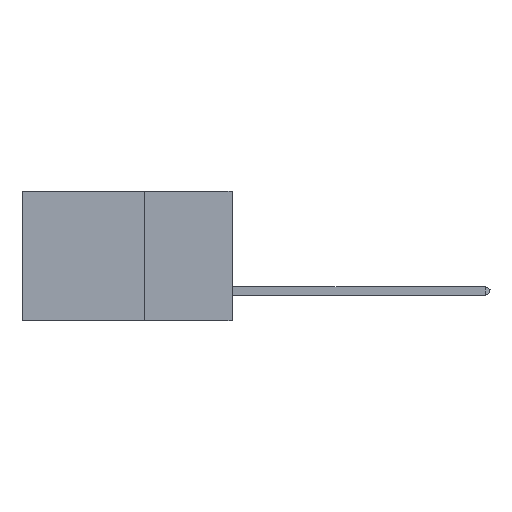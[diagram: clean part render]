
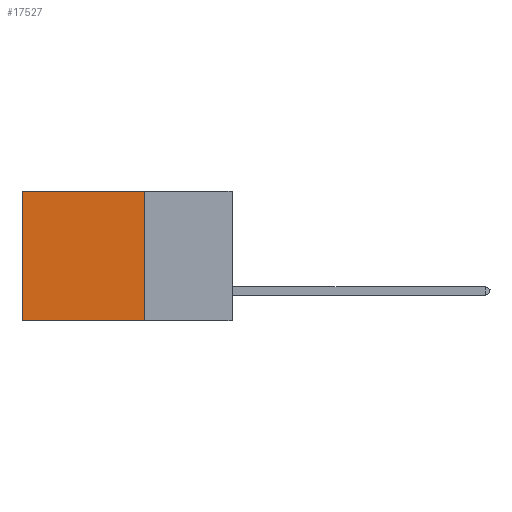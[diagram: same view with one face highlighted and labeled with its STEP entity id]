
A CAD part, left-side view. The second image highlights one B-rep face of the part: STEP entity #17527.
In plain terms, the highlighted planar face has unit normal (-1, 0, 0).
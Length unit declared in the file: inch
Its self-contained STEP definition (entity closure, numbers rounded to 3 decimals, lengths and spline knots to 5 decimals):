
#637 = CARTESIAN_POINT ( 'NONE',  ( 0.2875, 0.6, 0. ) ) ;
#1675 = VECTOR ( 'NONE', #4019, 39.37008 ) ;
#2315 = ORIENTED_EDGE ( 'NONE', *, *, #25332, .F. ) ;
#2528 = DIRECTION ( 'NONE',  ( 0., 1., 0. ) ) ;
#3520 = EDGE_CURVE ( 'NONE', #17088, #13766, #10512, .T. ) ;
#3753 = ORIENTED_EDGE ( 'NONE', *, *, #3520, .T. ) ;
#4019 = DIRECTION ( 'NONE',  ( 0., 1., 0. ) ) ;
#4047 = DIRECTION ( 'NONE',  ( 0., 0., -1. ) ) ;
#4694 = DIRECTION ( 'NONE',  ( 0., 0., -1. ) ) ;
#7903 = VECTOR ( 'NONE', #2528, 39.37008 ) ;
#8524 = VERTEX_POINT ( 'NONE', #17369 ) ;
#9736 = LINE ( 'NONE', #20987, #1675 ) ;
#10512 = LINE ( 'NONE', #12721, #28768 ) ;
#11515 = LINE ( 'NONE', #21692, #14612 ) ;
#12721 = CARTESIAN_POINT ( 'NONE',  ( 0.2875, 0.6, 0. ) ) ;
#13766 = VERTEX_POINT ( 'NONE', #29710 ) ;
#14612 = VECTOR ( 'NONE', #4694, 39.37008 ) ;
#16656 = FACE_OUTER_BOUND ( 'NONE', #34417, .T. ) ;
#17088 = VERTEX_POINT ( 'NONE', #637 ) ;
#17369 = CARTESIAN_POINT ( 'NONE',  ( 0.2875, 0.25, -0.37 ) ) ;
#17527 = ADVANCED_FACE ( 'NONE', ( #16656 ), #34238, .F. ) ;
#20165 = CARTESIAN_POINT ( 'NONE',  ( 0.2875, 0.25, 0. ) ) ;
#20987 = CARTESIAN_POINT ( 'NONE',  ( 0.2875, 0.25, 0. ) ) ;
#21692 = CARTESIAN_POINT ( 'NONE',  ( 0.2875, 0.25, 0. ) ) ;
#22951 = AXIS2_PLACEMENT_3D ( 'NONE', #20165, #29620, #4047 ) ;
#23052 = LINE ( 'NONE', #25108, #7903 ) ;
#25108 = CARTESIAN_POINT ( 'NONE',  ( 0.2875, 0.25, -0.37 ) ) ;
#25332 = EDGE_CURVE ( 'NONE', #31786, #8524, #11515, .T. ) ;
#26719 = DIRECTION ( 'NONE',  ( 0., 0., -1. ) ) ;
#26790 = ORIENTED_EDGE ( 'NONE', *, *, #33308, .T. ) ;
#28768 = VECTOR ( 'NONE', #26719, 39.37008 ) ;
#29620 = DIRECTION ( 'NONE',  ( 1., 0., 0. ) ) ;
#29710 = CARTESIAN_POINT ( 'NONE',  ( 0.2875, 0.6, -0.37 ) ) ;
#30263 = ORIENTED_EDGE ( 'NONE', *, *, #32347, .F. ) ;
#31786 = VERTEX_POINT ( 'NONE', #34904 ) ;
#32347 = EDGE_CURVE ( 'NONE', #8524, #13766, #23052, .T. ) ;
#33308 = EDGE_CURVE ( 'NONE', #31786, #17088, #9736, .T. ) ;
#34238 = PLANE ( 'NONE',  #22951 ) ;
#34417 = EDGE_LOOP ( 'NONE', ( #3753, #30263, #2315, #26790 ) ) ;
#34904 = CARTESIAN_POINT ( 'NONE',  ( 0.2875, 0.25, 0. ) ) ;
